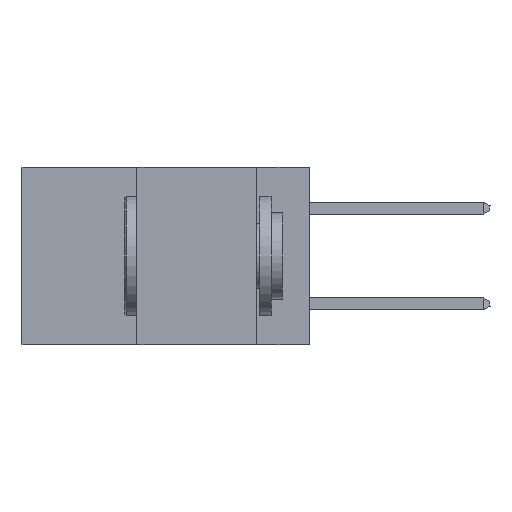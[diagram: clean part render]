
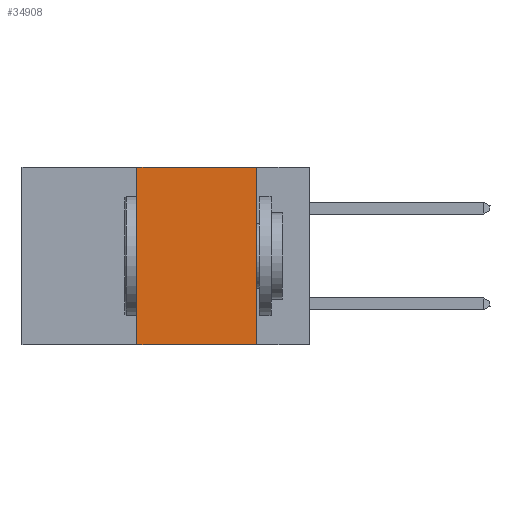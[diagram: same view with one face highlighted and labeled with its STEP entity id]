
A CAD part, left-side view. The second image highlights one B-rep face of the part: STEP entity #34908.
In plain terms, the highlighted planar face has unit normal (-1, 0, 0).
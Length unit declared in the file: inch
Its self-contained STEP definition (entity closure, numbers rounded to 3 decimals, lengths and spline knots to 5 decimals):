
#310 = ORIENTED_EDGE ( 'NONE', *, *, #3472, .F. ) ;
#2541 = ORIENTED_EDGE ( 'NONE', *, *, #27427, .T. ) ;
#2601 = DIRECTION ( 'NONE',  ( 1., 0., 0. ) ) ;
#2937 = EDGE_CURVE ( 'NONE', #34781, #37134, #4685, .T. ) ;
#3472 = EDGE_CURVE ( 'NONE', #14337, #25050, #23753, .T. ) ;
#3787 = ORIENTED_EDGE ( 'NONE', *, *, #2937, .F. ) ;
#4685 = LINE ( 'NONE', #27322, #10796 ) ;
#7974 = FACE_OUTER_BOUND ( 'NONE', #33655, .T. ) ;
#10796 = VECTOR ( 'NONE', #12584, 39.37008 ) ;
#12584 = DIRECTION ( 'NONE',  ( 0., 0., 1. ) ) ;
#14337 = VERTEX_POINT ( 'NONE', #19688 ) ;
#15859 = VECTOR ( 'NONE', #35409, 39.37008 ) ;
#17529 = PLANE ( 'NONE',  #36358 ) ;
#19688 = CARTESIAN_POINT ( 'NONE',  ( 0., 0.11, 0. ) ) ;
#21699 = VECTOR ( 'NONE', #27892, 39.37008 ) ;
#23523 = DIRECTION ( 'NONE',  ( 0., 0., -1. ) ) ;
#23712 = CARTESIAN_POINT ( 'NONE',  ( 0., 0.11, 0. ) ) ;
#23753 = LINE ( 'NONE', #23712, #15859 ) ;
#24923 = CARTESIAN_POINT ( 'NONE',  ( 0., 0.6, 0. ) ) ;
#25050 = VERTEX_POINT ( 'NONE', #27884 ) ;
#27322 = CARTESIAN_POINT ( 'NONE',  ( 0., 0.36, 0. ) ) ;
#27427 = EDGE_CURVE ( 'NONE', #34781, #25050, #35671, .T. ) ;
#27884 = CARTESIAN_POINT ( 'NONE',  ( 0., 0.11, -0.37 ) ) ;
#27892 = DIRECTION ( 'NONE',  ( 0., -1., 0. ) ) ;
#28931 = VECTOR ( 'NONE', #37058, 39.37008 ) ;
#30654 = EDGE_CURVE ( 'NONE', #37134, #14337, #37191, .T. ) ;
#31697 = ORIENTED_EDGE ( 'NONE', *, *, #30654, .F. ) ;
#33516 = CARTESIAN_POINT ( 'NONE',  ( 0., 0.36, 0. ) ) ;
#33655 = EDGE_LOOP ( 'NONE', ( #310, #31697, #3787, #2541 ) ) ;
#34187 = CARTESIAN_POINT ( 'NONE',  ( 0., 0.6, -0.37 ) ) ;
#34781 = VERTEX_POINT ( 'NONE', #37477 ) ;
#34908 = ADVANCED_FACE ( 'NONE', ( #7974 ), #17529, .F. ) ;
#35409 = DIRECTION ( 'NONE',  ( 0., 0., -1. ) ) ;
#35671 = LINE ( 'NONE', #34187, #28931 ) ;
#36358 = AXIS2_PLACEMENT_3D ( 'NONE', #37975, #2601, #23523 ) ;
#37058 = DIRECTION ( 'NONE',  ( 0., -1., 0. ) ) ;
#37134 = VERTEX_POINT ( 'NONE', #33516 ) ;
#37191 = LINE ( 'NONE', #24923, #21699 ) ;
#37477 = CARTESIAN_POINT ( 'NONE',  ( 0., 0.36, -0.37 ) ) ;
#37975 = CARTESIAN_POINT ( 'NONE',  ( 0., 0.6, 0. ) ) ;
